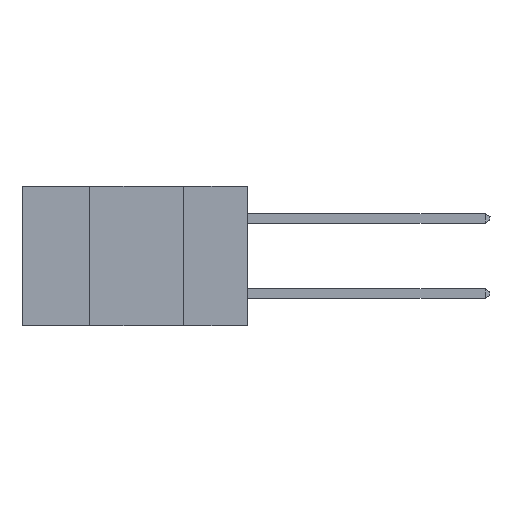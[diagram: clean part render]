
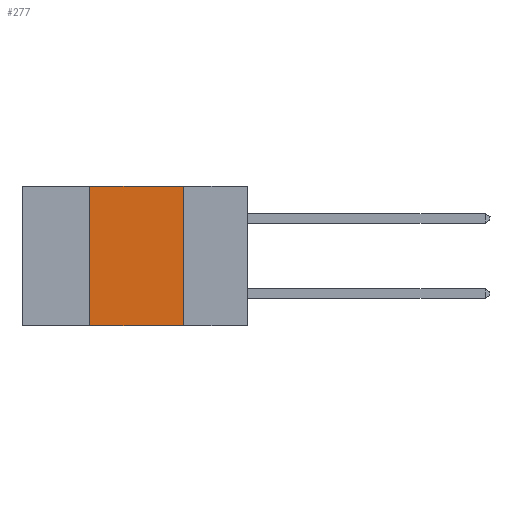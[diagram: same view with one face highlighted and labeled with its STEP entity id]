
A CAD part, left-side view. The second image highlights one B-rep face of the part: STEP entity #277.
In plain terms, the highlighted planar face has unit normal (-1, 0, 0).
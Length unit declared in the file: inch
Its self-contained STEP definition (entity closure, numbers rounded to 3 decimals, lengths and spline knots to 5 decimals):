
#277 = ADVANCED_FACE ( 'NONE', ( #10380 ), #12081, .F. ) ;
#1441 = VERTEX_POINT ( 'NONE', #14980 ) ;
#2202 = VERTEX_POINT ( 'NONE', #2933 ) ;
#2305 = EDGE_CURVE ( 'NONE', #9115, #1441, #5613, .T. ) ;
#2667 = DIRECTION ( 'NONE',  ( 0., -1., 0. ) ) ;
#2933 = CARTESIAN_POINT ( 'NONE',  ( 0., 0.17, -0.37 ) ) ;
#5613 = LINE ( 'NONE', #16999, #26775 ) ;
#6100 = ORIENTED_EDGE ( 'NONE', *, *, #2305, .F. ) ;
#6225 = VECTOR ( 'NONE', #2667, 39.37008 ) ;
#7086 = EDGE_CURVE ( 'NONE', #9115, #2202, #10326, .T. ) ;
#7988 = EDGE_CURVE ( 'NONE', #18364, #2202, #14585, .T. ) ;
#9020 = EDGE_CURVE ( 'NONE', #1441, #18364, #23135, .T. ) ;
#9115 = VERTEX_POINT ( 'NONE', #19913 ) ;
#9604 = VECTOR ( 'NONE', #18574, 39.37008 ) ;
#10326 = LINE ( 'NONE', #15746, #10988 ) ;
#10380 = FACE_OUTER_BOUND ( 'NONE', #13706, .T. ) ;
#10413 = ORIENTED_EDGE ( 'NONE', *, *, #7988, .F. ) ;
#10988 = VECTOR ( 'NONE', #17881, 39.37008 ) ;
#11114 = CARTESIAN_POINT ( 'NONE',  ( 0., 0.6, 0. ) ) ;
#11749 = ORIENTED_EDGE ( 'NONE', *, *, #7086, .T. ) ;
#12081 = PLANE ( 'NONE',  #18927 ) ;
#13706 = EDGE_LOOP ( 'NONE', ( #10413, #21675, #6100, #11749 ) ) ;
#14585 = LINE ( 'NONE', #20793, #9604 ) ;
#14980 = CARTESIAN_POINT ( 'NONE',  ( 0., 0.42, 0. ) ) ;
#15746 = CARTESIAN_POINT ( 'NONE',  ( 0., 0.6, -0.37 ) ) ;
#16999 = CARTESIAN_POINT ( 'NONE',  ( 0., 0.42, 0. ) ) ;
#17881 = DIRECTION ( 'NONE',  ( 0., -1., 0. ) ) ;
#18364 = VERTEX_POINT ( 'NONE', #25848 ) ;
#18574 = DIRECTION ( 'NONE',  ( 0., 0., -1. ) ) ;
#18927 = AXIS2_PLACEMENT_3D ( 'NONE', #22625, #25230, #25201 ) ;
#19913 = CARTESIAN_POINT ( 'NONE',  ( 0., 0.42, -0.37 ) ) ;
#20793 = CARTESIAN_POINT ( 'NONE',  ( 0., 0.17, 0. ) ) ;
#21675 = ORIENTED_EDGE ( 'NONE', *, *, #9020, .F. ) ;
#22625 = CARTESIAN_POINT ( 'NONE',  ( 0., 0.6, 0. ) ) ;
#23135 = LINE ( 'NONE', #11114, #6225 ) ;
#25201 = DIRECTION ( 'NONE',  ( 0., 0., -1. ) ) ;
#25230 = DIRECTION ( 'NONE',  ( 1., 0., 0. ) ) ;
#25572 = DIRECTION ( 'NONE',  ( 0., 0., 1. ) ) ;
#25848 = CARTESIAN_POINT ( 'NONE',  ( 0., 0.17, 0. ) ) ;
#26775 = VECTOR ( 'NONE', #25572, 39.37008 ) ;
